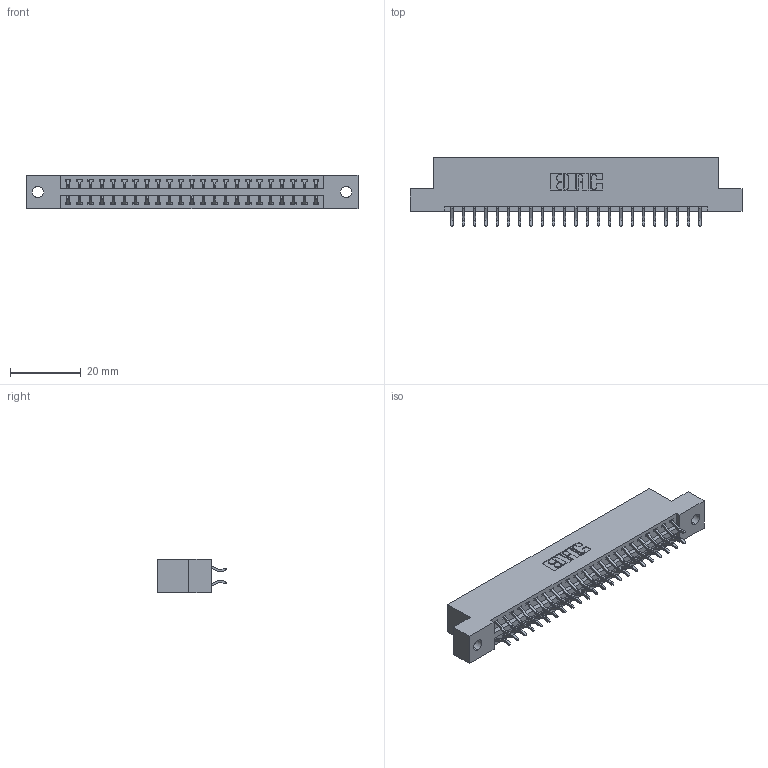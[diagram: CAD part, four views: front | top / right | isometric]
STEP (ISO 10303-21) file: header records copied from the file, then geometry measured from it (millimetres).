
FILE_DESCRIPTION (( 'STEP AP203' ), '1' );
FILE_NAME ('396-046-556-202.STEP', '2019-10-30T12:10:02', ( '' ), ( '' ), 'SwSTEP 2.0', 'SolidWorks 2016', '' );
FILE_SCHEMA (( 'CONFIG_CONTROL_DESIGN' ));
Length unit declared in the file: inch
Products named in the file (3): 396-046-556-202; 346 Part_Flush Mounting Lugs - 0.128 Dia; 345-292-001_556 Tail
Assembly tree (47 placements, depth 2):
  396-046-556-202
    346 Part_Flush Mounting Lugs - 0.128 Dia
    345-292-001_556 Tail  x46
Bounding box: 93.6 x 19.57 x 9.4 mm (x, y, z)
Volume: 8941 mm3; surface area: 11679.4 mm2
Topology: 47 solids, 47 shells, 2790 faces, 8287 edges, 5462 vertices
Faces by surface type: plane 1870, cylinder 920
Entity records: 17791 total; most frequent: CARTESIAN_POINT 2972, ORIENTED_EDGE 2894, DIRECTION 2659, EDGE_CURVE 1447, VECTOR 1215, LINE 1215, VERTEX_POINT 962, AXIS2_PLACEMENT_3D 722
